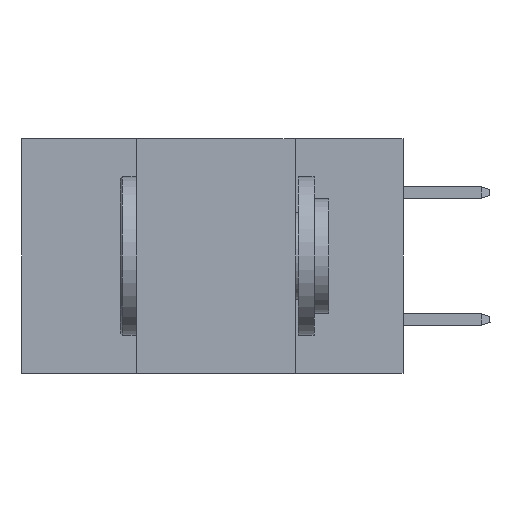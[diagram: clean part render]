
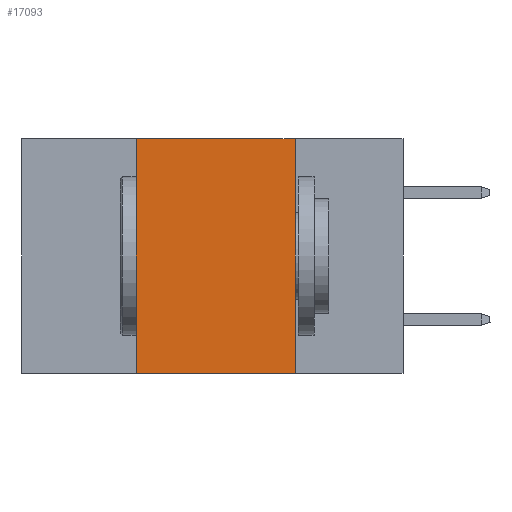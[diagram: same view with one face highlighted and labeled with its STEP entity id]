
A CAD part, left-side view. The second image highlights one B-rep face of the part: STEP entity #17093.
In plain terms, the highlighted planar face has unit normal (-1, 0, 0).
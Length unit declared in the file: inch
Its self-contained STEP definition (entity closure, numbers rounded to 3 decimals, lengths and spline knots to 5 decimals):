
#131 = FACE_OUTER_BOUND ( 'NONE', #18018, .T. ) ;
#233 = DIRECTION ( 'NONE',  ( 0., 0., -1. ) ) ;
#929 = DIRECTION ( 'NONE',  ( 0., -1., 0. ) ) ;
#1199 = VECTOR ( 'NONE', #21853, 39.37008 ) ;
#1799 = VERTEX_POINT ( 'NONE', #18324 ) ;
#2085 = CARTESIAN_POINT ( 'NONE',  ( 0., 0.6, 0. ) ) ;
#3815 = CARTESIAN_POINT ( 'NONE',  ( 0., 0.17, 0. ) ) ;
#5630 = DIRECTION ( 'NONE',  ( 0., 0., -1. ) ) ;
#5802 = EDGE_CURVE ( 'NONE', #18233, #1799, #7809, .T. ) ;
#6209 = CARTESIAN_POINT ( 'NONE',  ( 0., 0.42, 0. ) ) ;
#6585 = ORIENTED_EDGE ( 'NONE', *, *, #13012, .F. ) ;
#6808 = VECTOR ( 'NONE', #233, 39.37008 ) ;
#7090 = CARTESIAN_POINT ( 'NONE',  ( 0., 0.42, 0. ) ) ;
#7809 = LINE ( 'NONE', #7920, #6808 ) ;
#7885 = LINE ( 'NONE', #17665, #19883 ) ;
#7920 = CARTESIAN_POINT ( 'NONE',  ( 0., 0.17, 0. ) ) ;
#7986 = ORIENTED_EDGE ( 'NONE', *, *, #11082, .F. ) ;
#8814 = LINE ( 'NONE', #23322, #1199 ) ;
#9300 = DIRECTION ( 'NONE',  ( 1., 0., 0. ) ) ;
#11082 = EDGE_CURVE ( 'NONE', #19813, #14236, #15851, .T. ) ;
#13012 = EDGE_CURVE ( 'NONE', #14236, #18233, #7885, .T. ) ;
#13108 = ORIENTED_EDGE ( 'NONE', *, *, #5802, .F. ) ;
#14053 = EDGE_CURVE ( 'NONE', #19813, #1799, #8814, .T. ) ;
#14236 = VERTEX_POINT ( 'NONE', #7090 ) ;
#15851 = LINE ( 'NONE', #6209, #17455 ) ;
#16068 = AXIS2_PLACEMENT_3D ( 'NONE', #2085, #9300, #5630 ) ;
#17093 = ADVANCED_FACE ( 'NONE', ( #131 ), #22226, .F. ) ;
#17455 = VECTOR ( 'NONE', #17569, 39.37008 ) ;
#17569 = DIRECTION ( 'NONE',  ( 0., 0., 1. ) ) ;
#17665 = CARTESIAN_POINT ( 'NONE',  ( 0., 0.6, 0. ) ) ;
#18018 = EDGE_LOOP ( 'NONE', ( #13108, #6585, #7986, #22442 ) ) ;
#18233 = VERTEX_POINT ( 'NONE', #3815 ) ;
#18324 = CARTESIAN_POINT ( 'NONE',  ( 0., 0.17, -0.37 ) ) ;
#19813 = VERTEX_POINT ( 'NONE', #21137 ) ;
#19883 = VECTOR ( 'NONE', #929, 39.37008 ) ;
#21137 = CARTESIAN_POINT ( 'NONE',  ( 0., 0.42, -0.37 ) ) ;
#21853 = DIRECTION ( 'NONE',  ( 0., -1., 0. ) ) ;
#22226 = PLANE ( 'NONE',  #16068 ) ;
#22442 = ORIENTED_EDGE ( 'NONE', *, *, #14053, .T. ) ;
#23322 = CARTESIAN_POINT ( 'NONE',  ( 0., 0.6, -0.37 ) ) ;
